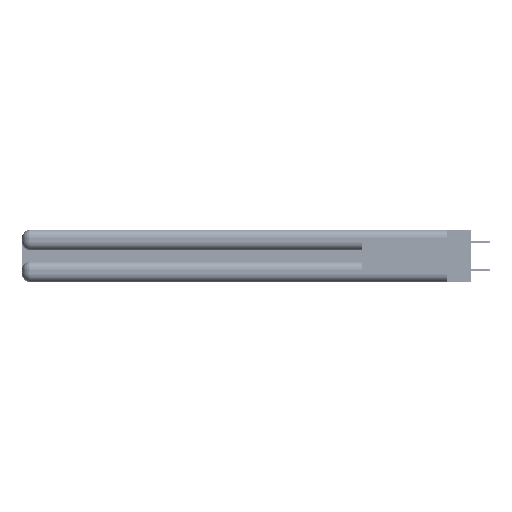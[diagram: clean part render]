
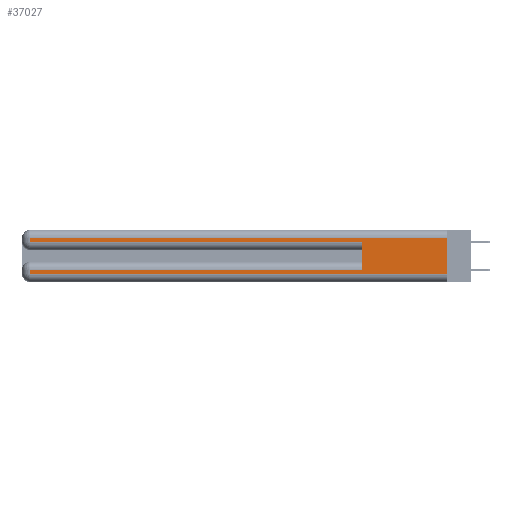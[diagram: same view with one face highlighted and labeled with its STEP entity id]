
A CAD part, left-side view. The second image highlights one B-rep face of the part: STEP entity #37027.
In plain terms, the highlighted planar face has unit normal (-1, 0, 0).
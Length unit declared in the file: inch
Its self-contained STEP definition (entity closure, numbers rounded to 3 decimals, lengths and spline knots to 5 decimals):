
#9 = LINE ( 'NONE', #51228, #11307 ) ;
#209 = LINE ( 'NONE', #18373, #53211 ) ;
#534 = CARTESIAN_POINT ( 'NONE',  ( 0., 0., 0.06 ) ) ;
#540 = CARTESIAN_POINT ( 'NONE',  ( 0., 0., 0.31 ) ) ;
#1311 = LINE ( 'NONE', #39117, #2211 ) ;
#1648 = AXIS2_PLACEMENT_3D ( 'NONE', #45545, #45273, #2151 ) ;
#2151 = DIRECTION ( 'NONE',  ( 0., 0., -1. ) ) ;
#2211 = VECTOR ( 'NONE', #51999, 39.37008 ) ;
#2854 = CARTESIAN_POINT ( 'NONE',  ( 0., 0., 0.085 ) ) ;
#5334 = EDGE_LOOP ( 'NONE', ( #9240, #45443, #8738, #35039, #12498, #16717, #11242, #27325 ) ) ;
#5337 = LINE ( 'NONE', #22695, #8936 ) ;
#5465 = CARTESIAN_POINT ( 'NONE',  ( 0., 2.94, 0.06 ) ) ;
#6101 = CARTESIAN_POINT ( 'NONE',  ( 0., 2.94, 0.31 ) ) ;
#8738 = ORIENTED_EDGE ( 'NONE', *, *, #36785, .T. ) ;
#8936 = VECTOR ( 'NONE', #35862, 39.37008 ) ;
#9065 = VERTEX_POINT ( 'NONE', #540 ) ;
#9240 = ORIENTED_EDGE ( 'NONE', *, *, #34222, .F. ) ;
#11242 = ORIENTED_EDGE ( 'NONE', *, *, #35030, .T. ) ;
#11307 = VECTOR ( 'NONE', #12855, 39.37008 ) ;
#12498 = ORIENTED_EDGE ( 'NONE', *, *, #45853, .F. ) ;
#12855 = DIRECTION ( 'NONE',  ( 0., 0., -1. ) ) ;
#16717 = ORIENTED_EDGE ( 'NONE', *, *, #53758, .T. ) ;
#17393 = CARTESIAN_POINT ( 'NONE',  ( 0., 0.6, 0.085 ) ) ;
#18373 = CARTESIAN_POINT ( 'NONE',  ( 0., 0., 0.285 ) ) ;
#18579 = DIRECTION ( 'NONE',  ( 0., 0., -1. ) ) ;
#18582 = VECTOR ( 'NONE', #35477, 39.37008 ) ;
#18950 = PLANE ( 'NONE',  #1648 ) ;
#19073 = VERTEX_POINT ( 'NONE', #44860 ) ;
#21050 = VERTEX_POINT ( 'NONE', #534 ) ;
#22695 = CARTESIAN_POINT ( 'NONE',  ( 0., 0.6, 0.145 ) ) ;
#25807 = EDGE_CURVE ( 'NONE', #9065, #42006, #54035, .T. ) ;
#26244 = LINE ( 'NONE', #27362, #18582 ) ;
#26439 = EDGE_CURVE ( 'NONE', #19073, #48473, #209, .T. ) ;
#27325 = ORIENTED_EDGE ( 'NONE', *, *, #30259, .T. ) ;
#27362 = CARTESIAN_POINT ( 'NONE',  ( 0., 2.94, 0.37 ) ) ;
#28192 = FACE_OUTER_BOUND ( 'NONE', #5334, .T. ) ;
#30259 = EDGE_CURVE ( 'NONE', #45508, #21050, #1311, .T. ) ;
#30637 = CARTESIAN_POINT ( 'NONE',  ( 0., 0., 0.37 ) ) ;
#30985 = DIRECTION ( 'NONE',  ( 0., -1., 0. ) ) ;
#31389 = CARTESIAN_POINT ( 'NONE',  ( 0., 2.94, 0.085 ) ) ;
#32215 = CARTESIAN_POINT ( 'NONE',  ( 0., 0., 0.31 ) ) ;
#33086 = DIRECTION ( 'NONE',  ( 0., 1., 0. ) ) ;
#34222 = EDGE_CURVE ( 'NONE', #9065, #21050, #51913, .T. ) ;
#35030 = EDGE_CURVE ( 'NONE', #38614, #45508, #9, .T. ) ;
#35039 = ORIENTED_EDGE ( 'NONE', *, *, #26439, .T. ) ;
#35477 = DIRECTION ( 'NONE',  ( 0., 0., -1. ) ) ;
#35862 = DIRECTION ( 'NONE',  ( 0., 0., 1. ) ) ;
#36137 = DIRECTION ( 'NONE',  ( 0., 1., 0. ) ) ;
#36785 = EDGE_CURVE ( 'NONE', #42006, #19073, #26244, .T. ) ;
#37027 = ADVANCED_FACE ( 'NONE', ( #28192 ), #18950, .F. ) ;
#38227 = CARTESIAN_POINT ( 'NONE',  ( 0., 0.6, 0.285 ) ) ;
#38523 = VERTEX_POINT ( 'NONE', #17393 ) ;
#38614 = VERTEX_POINT ( 'NONE', #31389 ) ;
#39117 = CARTESIAN_POINT ( 'NONE',  ( 0., 0., 0.06 ) ) ;
#39843 = VECTOR ( 'NONE', #33086, 39.37008 ) ;
#41214 = LINE ( 'NONE', #2854, #39843 ) ;
#42006 = VERTEX_POINT ( 'NONE', #6101 ) ;
#44860 = CARTESIAN_POINT ( 'NONE',  ( 0., 2.94, 0.285 ) ) ;
#45263 = VECTOR ( 'NONE', #18579, 39.37008 ) ;
#45273 = DIRECTION ( 'NONE',  ( 1., 0., 0. ) ) ;
#45443 = ORIENTED_EDGE ( 'NONE', *, *, #25807, .T. ) ;
#45508 = VERTEX_POINT ( 'NONE', #5465 ) ;
#45545 = CARTESIAN_POINT ( 'NONE',  ( 0., 0., 0.37 ) ) ;
#45853 = EDGE_CURVE ( 'NONE', #38523, #48473, #5337, .T. ) ;
#48473 = VERTEX_POINT ( 'NONE', #38227 ) ;
#49735 = VECTOR ( 'NONE', #36137, 39.37008 ) ;
#51228 = CARTESIAN_POINT ( 'NONE',  ( 0., 2.94, 0.37 ) ) ;
#51913 = LINE ( 'NONE', #30637, #45263 ) ;
#51999 = DIRECTION ( 'NONE',  ( 0., -1., 0. ) ) ;
#53211 = VECTOR ( 'NONE', #30985, 39.37008 ) ;
#53758 = EDGE_CURVE ( 'NONE', #38523, #38614, #41214, .T. ) ;
#54035 = LINE ( 'NONE', #32215, #49735 ) ;
